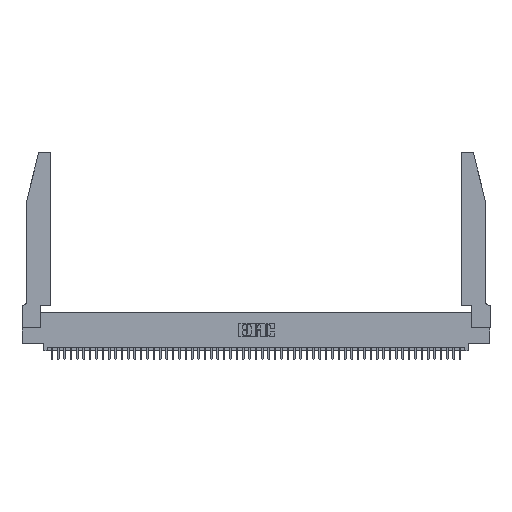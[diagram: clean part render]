
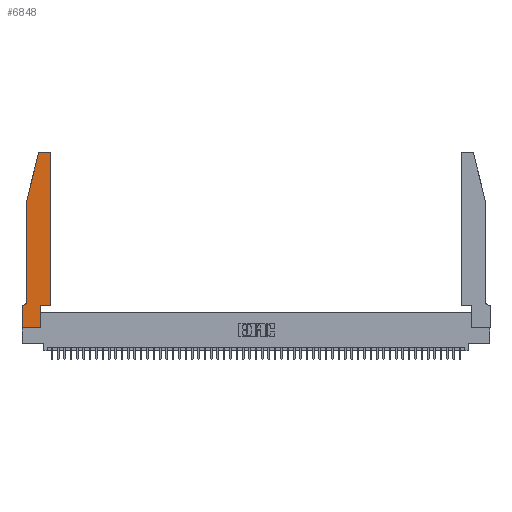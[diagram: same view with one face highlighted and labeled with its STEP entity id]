
A CAD part, top view. The second image highlights one B-rep face of the part: STEP entity #6848.
In plain terms, the highlighted planar face has unit normal (0, 0, 1).
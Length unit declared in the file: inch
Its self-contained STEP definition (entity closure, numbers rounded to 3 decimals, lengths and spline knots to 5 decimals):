
#384 = DIRECTION ( 'NONE',  ( -0.239, -0.971, 0. ) ) ;
#1106 = DIRECTION ( 'NONE',  ( 0., 0., -1. ) ) ;
#2392 = EDGE_LOOP ( 'NONE', ( #25482, #47868, #27502, #46892, #9266, #37638, #38816, #12129, #38952, #2608, #45384, #2824 ) ) ;
#2608 = ORIENTED_EDGE ( 'NONE', *, *, #20899, .T. ) ;
#2824 = ORIENTED_EDGE ( 'NONE', *, *, #29904, .T. ) ;
#2846 = CARTESIAN_POINT ( 'NONE',  ( 0.4505, 2.72, 0.37 ) ) ;
#3498 = DIRECTION ( 'NONE',  ( 0., 1., 0. ) ) ;
#3789 = EDGE_CURVE ( 'NONE', #39184, #24269, #8209, .T. ) ;
#4083 = VERTEX_POINT ( 'NONE', #6177 ) ;
#5701 = CARTESIAN_POINT ( 'NONE',  ( 0., 0.35, 0.37 ) ) ;
#5854 = DIRECTION ( 'NONE',  ( 0., 0., 1. ) ) ;
#6061 = EDGE_CURVE ( 'NONE', #43577, #4083, #38630, .T. ) ;
#6177 = CARTESIAN_POINT ( 'NONE',  ( 0.0055, 0.35, 0.37 ) ) ;
#6848 = ADVANCED_FACE ( 'NONE', ( #15005 ), #46383, .T. ) ;
#8209 = LINE ( 'NONE', #8380, #28607 ) ;
#8380 = CARTESIAN_POINT ( 'NONE',  ( 0.2605, 2.75, 0.37 ) ) ;
#8473 = DIRECTION ( 'NONE',  ( 0., 1., 0. ) ) ;
#9204 = LINE ( 'NONE', #28495, #50020 ) ;
#9208 = EDGE_CURVE ( 'NONE', #24269, #52289, #9657, .T. ) ;
#9266 = ORIENTED_EDGE ( 'NONE', *, *, #6061, .T. ) ;
#9657 = CIRCLE ( 'NONE', #34931, 0.03 ) ;
#9842 = DIRECTION ( 'NONE',  ( 1., 0., 0. ) ) ;
#10407 = EDGE_CURVE ( 'NONE', #4083, #28944, #52240, .T. ) ;
#11070 = VECTOR ( 'NONE', #49303, 39.37008 ) ;
#11864 = VECTOR ( 'NONE', #3498, 39.37008 ) ;
#12129 = ORIENTED_EDGE ( 'NONE', *, *, #47270, .T. ) ;
#12200 = DIRECTION ( 'NONE',  ( 0., -1., 0. ) ) ;
#12290 = VERTEX_POINT ( 'NONE', #2846 ) ;
#12622 = CARTESIAN_POINT ( 'NONE',  ( 0.0755, 2., 0.37 ) ) ;
#14223 = VERTEX_POINT ( 'NONE', #28341 ) ;
#14924 = DIRECTION ( 'NONE',  ( -1., 0., 0. ) ) ;
#15005 = FACE_OUTER_BOUND ( 'NONE', #2392, .T. ) ;
#15200 = DIRECTION ( 'NONE',  ( 0., 0., 1. ) ) ;
#15282 = VECTOR ( 'NONE', #8473, 39.37008 ) ;
#16210 = VERTEX_POINT ( 'NONE', #41314 ) ;
#17207 = VECTOR ( 'NONE', #12200, 39.37008 ) ;
#18631 = CARTESIAN_POINT ( 'NONE',  ( 0.284, 2.75, 0.37 ) ) ;
#19544 = AXIS2_PLACEMENT_3D ( 'NONE', #25629, #1106, #29698 ) ;
#19799 = VECTOR ( 'NONE', #14924, 39.37008 ) ;
#20663 = CARTESIAN_POINT ( 'NONE',  ( 0.2865, 0.35, 0.37 ) ) ;
#20687 = AXIS2_PLACEMENT_3D ( 'NONE', #30323, #5854, #34398 ) ;
#20899 = EDGE_CURVE ( 'NONE', #48943, #14223, #32702, .T. ) ;
#22730 = LINE ( 'NONE', #23904, #11864 ) ;
#23904 = CARTESIAN_POINT ( 'NONE',  ( 0.4505, 0.35, 0.37 ) ) ;
#24269 = VERTEX_POINT ( 'NONE', #18631 ) ;
#24553 = CARTESIAN_POINT ( 'NONE',  ( 0.4205, 2.75, 0.37 ) ) ;
#25047 = VERTEX_POINT ( 'NONE', #51816 ) ;
#25482 = ORIENTED_EDGE ( 'NONE', *, *, #3789, .T. ) ;
#25629 = CARTESIAN_POINT ( 'NONE',  ( 0.0055, 0.42, 0.37 ) ) ;
#25668 = DIRECTION ( 'NONE',  ( 1., 0., 0. ) ) ;
#26128 = LINE ( 'NONE', #20663, #15282 ) ;
#27261 = LINE ( 'NONE', #12622, #36768 ) ;
#27502 = ORIENTED_EDGE ( 'NONE', *, *, #46068, .T. ) ;
#28341 = CARTESIAN_POINT ( 'NONE',  ( 0.4505, 0.35, 0.37 ) ) ;
#28495 = CARTESIAN_POINT ( 'NONE',  ( 0., 0., 0.37 ) ) ;
#28607 = VECTOR ( 'NONE', #40973, 39.37008 ) ;
#28944 = VERTEX_POINT ( 'NONE', #52319 ) ;
#29698 = DIRECTION ( 'NONE',  ( -1., 0., 0. ) ) ;
#29904 = EDGE_CURVE ( 'NONE', #12290, #39184, #48611, .T. ) ;
#30323 = CARTESIAN_POINT ( 'NONE',  ( 0.4205, 2.72, 0.37 ) ) ;
#30504 = CARTESIAN_POINT ( 'NONE',  ( 0.2865, 0.35, 0.37 ) ) ;
#30607 = LINE ( 'NONE', #40637, #17207 ) ;
#30938 = VERTEX_POINT ( 'NONE', #36983 ) ;
#30958 = CARTESIAN_POINT ( 'NONE',  ( 0.25487, 2.72718, 0.37 ) ) ;
#31122 = CARTESIAN_POINT ( 'NONE',  ( 0.0755, 0.35, 0.37 ) ) ;
#31920 = EDGE_CURVE ( 'NONE', #30938, #43577, #30607, .T. ) ;
#32702 = LINE ( 'NONE', #36972, #11070 ) ;
#34196 = LINE ( 'NONE', #50041, #43759 ) ;
#34240 = DIRECTION ( 'NONE',  ( 0., 0., 1. ) ) ;
#34268 = EDGE_CURVE ( 'NONE', #28944, #16210, #9204, .T. ) ;
#34398 = DIRECTION ( 'NONE',  ( 1., 0., 0. ) ) ;
#34931 = AXIS2_PLACEMENT_3D ( 'NONE', #39563, #15200, #43672 ) ;
#36768 = VECTOR ( 'NONE', #384, 39.37008 ) ;
#36972 = CARTESIAN_POINT ( 'NONE',  ( 0.4505, 0.35, 0.37 ) ) ;
#36983 = CARTESIAN_POINT ( 'NONE',  ( 0.0755, 2., 0.37 ) ) ;
#37638 = ORIENTED_EDGE ( 'NONE', *, *, #10407, .T. ) ;
#38630 = CIRCLE ( 'NONE', #19544, 0.07 ) ;
#38816 = ORIENTED_EDGE ( 'NONE', *, *, #34268, .T. ) ;
#38952 = ORIENTED_EDGE ( 'NONE', *, *, #44053, .T. ) ;
#39184 = VERTEX_POINT ( 'NONE', #24553 ) ;
#39563 = CARTESIAN_POINT ( 'NONE',  ( 0.284, 2.72, 0.37 ) ) ;
#40484 = EDGE_CURVE ( 'NONE', #14223, #12290, #22730, .T. ) ;
#40637 = CARTESIAN_POINT ( 'NONE',  ( 0.0755, 2., 0.37 ) ) ;
#40973 = DIRECTION ( 'NONE',  ( -1., 0., 0. ) ) ;
#41314 = CARTESIAN_POINT ( 'NONE',  ( 0., 0., 0.37 ) ) ;
#43577 = VERTEX_POINT ( 'NONE', #45193 ) ;
#43672 = DIRECTION ( 'NONE',  ( 1., 0., 0. ) ) ;
#43759 = VECTOR ( 'NONE', #25668, 39.37008 ) ;
#44053 = EDGE_CURVE ( 'NONE', #25047, #48943, #26128, .T. ) ;
#44715 = DIRECTION ( 'NONE',  ( 0., -1., 0. ) ) ;
#45193 = CARTESIAN_POINT ( 'NONE',  ( 0.0755, 0.42, 0.37 ) ) ;
#45384 = ORIENTED_EDGE ( 'NONE', *, *, #40484, .T. ) ;
#46068 = EDGE_CURVE ( 'NONE', #52289, #30938, #27261, .T. ) ;
#46383 = PLANE ( 'NONE',  #47530 ) ;
#46892 = ORIENTED_EDGE ( 'NONE', *, *, #31920, .T. ) ;
#47270 = EDGE_CURVE ( 'NONE', #16210, #25047, #34196, .T. ) ;
#47530 = AXIS2_PLACEMENT_3D ( 'NONE', #5701, #34240, #9842 ) ;
#47868 = ORIENTED_EDGE ( 'NONE', *, *, #9208, .T. ) ;
#48611 = CIRCLE ( 'NONE', #20687, 0.03 ) ;
#48943 = VERTEX_POINT ( 'NONE', #30504 ) ;
#49303 = DIRECTION ( 'NONE',  ( 1., 0., 0. ) ) ;
#50020 = VECTOR ( 'NONE', #44715, 39.37008 ) ;
#50041 = CARTESIAN_POINT ( 'NONE',  ( 0., 0., 0.37 ) ) ;
#51816 = CARTESIAN_POINT ( 'NONE',  ( 0.2865, 0., 0.37 ) ) ;
#52240 = LINE ( 'NONE', #31122, #19799 ) ;
#52289 = VERTEX_POINT ( 'NONE', #30958 ) ;
#52319 = CARTESIAN_POINT ( 'NONE',  ( 0., 0.35, 0.37 ) ) ;
